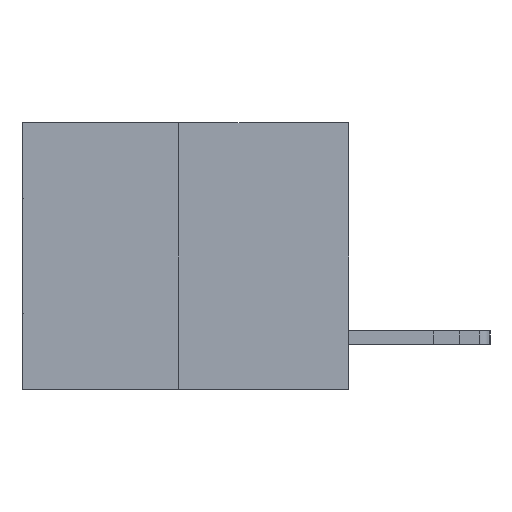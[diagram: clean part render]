
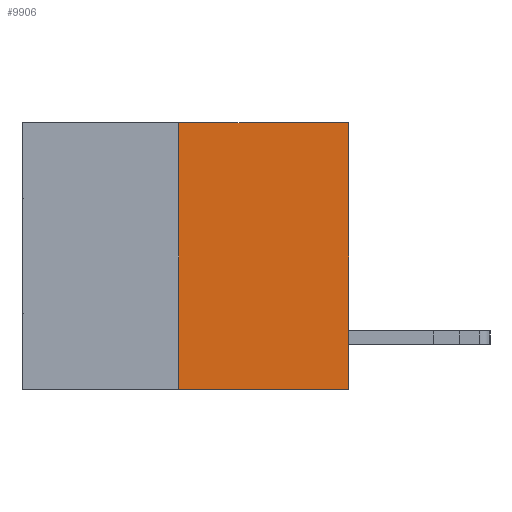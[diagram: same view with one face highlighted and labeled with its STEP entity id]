
A CAD part, left-side view. The second image highlights one B-rep face of the part: STEP entity #9906.
In plain terms, the highlighted planar face has unit normal (-1, 0, 0).
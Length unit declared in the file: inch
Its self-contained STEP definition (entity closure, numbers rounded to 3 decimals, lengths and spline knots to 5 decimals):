
#1301 = FACE_OUTER_BOUND ( 'NONE', #14025, .T. ) ;
#2094 = DIRECTION ( 'NONE',  ( 0., 0., 1. ) ) ;
#2292 = VECTOR ( 'NONE', #17861, 39.37008 ) ;
#2808 = LINE ( 'NONE', #10278, #29934 ) ;
#2818 = PLANE ( 'NONE',  #28804 ) ;
#3071 = LINE ( 'NONE', #25201, #2292 ) ;
#3484 = DIRECTION ( 'NONE',  ( 0., -1., 0. ) ) ;
#4085 = ORIENTED_EDGE ( 'NONE', *, *, #25936, .F. ) ;
#4325 = EDGE_CURVE ( 'NONE', #23431, #19891, #5058, .T. ) ;
#5058 = LINE ( 'NONE', #15692, #9305 ) ;
#5326 = CARTESIAN_POINT ( 'NONE',  ( 0., 0.6, 0. ) ) ;
#7711 = CARTESIAN_POINT ( 'NONE',  ( 0., 0., -0.49 ) ) ;
#7797 = DIRECTION ( 'NONE',  ( 1., 0., 0. ) ) ;
#8725 = ORIENTED_EDGE ( 'NONE', *, *, #29308, .T. ) ;
#9305 = VECTOR ( 'NONE', #3484, 39.37008 ) ;
#9906 = ADVANCED_FACE ( 'NONE', ( #1301 ), #2818, .F. ) ;
#10278 = CARTESIAN_POINT ( 'NONE',  ( 0., 0., 0. ) ) ;
#10777 = ORIENTED_EDGE ( 'NONE', *, *, #4325, .F. ) ;
#11254 = ORIENTED_EDGE ( 'NONE', *, *, #16245, .T. ) ;
#14025 = EDGE_LOOP ( 'NONE', ( #4085, #8725, #11254, #10777 ) ) ;
#14873 = VERTEX_POINT ( 'NONE', #7711 ) ;
#15272 = CARTESIAN_POINT ( 'NONE',  ( 0., 0.312, 0. ) ) ;
#15692 = CARTESIAN_POINT ( 'NONE',  ( 0., 0.6, 0. ) ) ;
#16245 = EDGE_CURVE ( 'NONE', #14873, #19891, #2808, .T. ) ;
#16425 = VECTOR ( 'NONE', #2094, 39.37008 ) ;
#16805 = CARTESIAN_POINT ( 'NONE',  ( 0., 0.312, -0.49 ) ) ;
#17861 = DIRECTION ( 'NONE',  ( 0., -1., 0. ) ) ;
#17879 = DIRECTION ( 'NONE',  ( 0., 0., 1. ) ) ;
#18006 = CARTESIAN_POINT ( 'NONE',  ( 0., 0., 0. ) ) ;
#19891 = VERTEX_POINT ( 'NONE', #18006 ) ;
#20676 = VERTEX_POINT ( 'NONE', #29354 ) ;
#23431 = VERTEX_POINT ( 'NONE', #15272 ) ;
#24185 = LINE ( 'NONE', #16805, #16425 ) ;
#25201 = CARTESIAN_POINT ( 'NONE',  ( 0., 0.6, -0.49 ) ) ;
#25936 = EDGE_CURVE ( 'NONE', #20676, #23431, #24185, .T. ) ;
#28804 = AXIS2_PLACEMENT_3D ( 'NONE', #5326, #7797, #30102 ) ;
#29308 = EDGE_CURVE ( 'NONE', #20676, #14873, #3071, .T. ) ;
#29354 = CARTESIAN_POINT ( 'NONE',  ( 0., 0.312, -0.49 ) ) ;
#29934 = VECTOR ( 'NONE', #17879, 39.37008 ) ;
#30102 = DIRECTION ( 'NONE',  ( 0., 0., -1. ) ) ;
